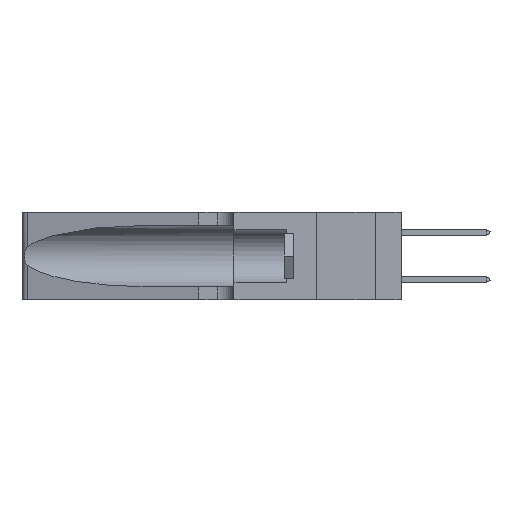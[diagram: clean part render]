
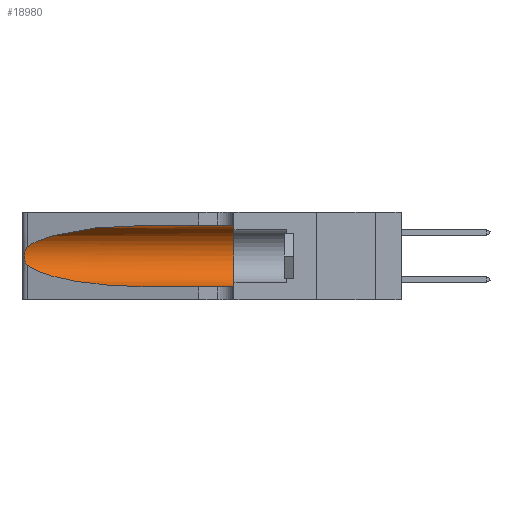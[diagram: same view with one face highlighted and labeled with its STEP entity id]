
A CAD part, left-side view. The second image highlights one B-rep face of the part: STEP entity #18980.
In plain terms, the highlighted cylindrical face has radius 3.308 mm (diameter 6.617 mm), a partial arc.
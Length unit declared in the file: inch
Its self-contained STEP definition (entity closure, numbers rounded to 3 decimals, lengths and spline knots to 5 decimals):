
#847 = CARTESIAN_POINT ( 'NONE',  ( 0.26075, 1.23896, 0.178 ) ) ;
#1594 = B_SPLINE_CURVE_WITH_KNOTS ( 'NONE', 3,
 ( #9400, #29070, #12274, #31901, #15130, #34700, #17978, #847, #20798, #3743, #23626, #6642, #26400, #9530 ),
 .UNSPECIFIED., .F., .F.,
 ( 4, 2, 2, 2, 2, 2, 4 ),
 ( 0., 0.00027, 0.00053, 0.00107, 0.0016, 0.00187, 0.00214 ),
 .UNSPECIFIED. ) ;
#2222 = DIRECTION ( 'NONE',  ( 0., 1., 0. ) ) ;
#2619 = CARTESIAN_POINT ( 'NONE',  ( 0.25487, 1.22718, 0.14631 ) ) ;
#3743 = CARTESIAN_POINT ( 'NONE',  ( 0.25856, 1.23593, 0.16098 ) ) ;
#4929 = LINE ( 'NONE', #19138, #19169 ) ;
#4961 = DIRECTION ( 'NONE',  ( 0., -1., 0. ) ) ;
#5533 =( BOUNDED_CURVE ( )  B_SPLINE_CURVE ( 3, ( #9325, #23425, #15048, #34634 ),
 .UNSPECIFIED., .F., .T. ) 
 B_SPLINE_CURVE_WITH_KNOTS ( ( 4, 4 ),
 ( 3.44316, 4.71239 ),
 .UNSPECIFIED. ) 
 CURVE ( )  GEOMETRIC_REPRESENTATION_ITEM ( )  RATIONAL_B_SPLINE_CURVE ( ( 1., 0.87, 0.87, 1. ) ) 
 REPRESENTATION_ITEM ( '' )  );
#6642 = CARTESIAN_POINT ( 'NONE',  ( 0.25639, 1.23186, 0.15144 ) ) ;
#6939 = CARTESIAN_POINT ( 'NONE',  ( 0.2373, 1.15595, 0.28018 ) ) ;
#7220 = DIRECTION ( 'NONE',  ( 0., -1., 0. ) ) ;
#7723 = AXIS2_PLACEMENT_3D ( 'NONE', #32463, #7220, #26968 ) ;
#7843 = VERTEX_POINT ( 'NONE', #20729 ) ;
#8729 = VERTEX_POINT ( 'NONE', #20618 ) ;
#9325 = CARTESIAN_POINT ( 'NONE',  ( 0.25487, 1.22718, 0.14631 ) ) ;
#9400 = CARTESIAN_POINT ( 'NONE',  ( 0.25487, 1.22718, 0.22369 ) ) ;
#9530 = CARTESIAN_POINT ( 'NONE',  ( 0.25487, 1.22718, 0.14631 ) ) ;
#9717 = CARTESIAN_POINT ( 'NONE',  ( 0.1305, 0.72297, 0.31525 ) ) ;
#12274 = CARTESIAN_POINT ( 'NONE',  ( 0.25639, 1.23184, 0.21858 ) ) ;
#15048 = CARTESIAN_POINT ( 'NONE',  ( 0.18966, 0.96281, 0.05475 ) ) ;
#15130 = CARTESIAN_POINT ( 'NONE',  ( 0.25854, 1.2359, 0.20912 ) ) ;
#16181 = DIRECTION ( 'NONE',  ( 0., -1., 0. ) ) ;
#17978 = CARTESIAN_POINT ( 'NONE',  ( 0.26075, 1.23896, 0.19203 ) ) ;
#18260 = CARTESIAN_POINT ( 'NONE',  ( 0.18966, 0.96281, 0.31525 ) ) ;
#18316 = VERTEX_POINT ( 'NONE', #29688 ) ;
#18980 = ADVANCED_FACE ( 'NONE', ( #30501 ), #22222, .F. ) ;
#19138 = CARTESIAN_POINT ( 'NONE',  ( 0.1305, 1.61858, 0.31525 ) ) ;
#19169 = VECTOR ( 'NONE', #4961, 39.37008 ) ;
#19300 = CARTESIAN_POINT ( 'NONE',  ( 0.1305, 0.35, 0.185 ) ) ;
#20207 = EDGE_CURVE ( 'NONE', #8729, #27805, #1594, .T. ) ;
#20618 = CARTESIAN_POINT ( 'NONE',  ( 0.25487, 1.22718, 0.22369 ) ) ;
#20729 = CARTESIAN_POINT ( 'NONE',  ( 0.1305, 0.72297, 0.05475 ) ) ;
#20798 = CARTESIAN_POINT ( 'NONE',  ( 0.26017, 1.23833, 0.17102 ) ) ;
#20882 = ORIENTED_EDGE ( 'NONE', *, *, #26905, .T. ) ;
#21963 = ORIENTED_EDGE ( 'NONE', *, *, #30637, .T. ) ;
#21986 = ORIENTED_EDGE ( 'NONE', *, *, #20207, .T. ) ;
#22128 = DIRECTION ( 'NONE',  ( 0., 0., 1. ) ) ;
#22222 = CYLINDRICAL_SURFACE ( 'NONE', #7723, 0.13025 ) ;
#23425 = CARTESIAN_POINT ( 'NONE',  ( 0.2373, 1.15595, 0.08982 ) ) ;
#23626 = CARTESIAN_POINT ( 'NONE',  ( 0.25789, 1.23486, 0.15765 ) ) ;
#24091 = VERTEX_POINT ( 'NONE', #27005 ) ;
#24323 = ORIENTED_EDGE ( 'NONE', *, *, #26958, .F. ) ;
#25141 = EDGE_CURVE ( 'NONE', #27805, #7843, #5533, .T. ) ;
#26400 = CARTESIAN_POINT ( 'NONE',  ( 0.25555, 1.22993, 0.14849 ) ) ;
#26703 = CARTESIAN_POINT ( 'NONE',  ( 0.25487, 1.22718, 0.22369 ) ) ;
#26905 = EDGE_CURVE ( 'NONE', #7843, #24091, #28328, .T. ) ;
#26958 = EDGE_CURVE ( 'NONE', #18316, #31938, #4929, .T. ) ;
#26968 = DIRECTION ( 'NONE',  ( 0., 0., -1. ) ) ;
#27005 = CARTESIAN_POINT ( 'NONE',  ( 0.1305, 0.35, 0.05475 ) ) ;
#27805 = VERTEX_POINT ( 'NONE', #2619 ) ;
#27815 = EDGE_LOOP ( 'NONE', ( #21963, #21986, #35365, #20882, #35640, #24323 ) ) ;
#28328 = LINE ( 'NONE', #35726, #31844 ) ;
#29043 =( BOUNDED_CURVE ( )  B_SPLINE_CURVE ( 3, ( #9717, #18260, #6939, #26703 ),
 .UNSPECIFIED., .F., .T. ) 
 B_SPLINE_CURVE_WITH_KNOTS ( ( 4, 4 ),
 ( 1.5708, 2.84003 ),
 .UNSPECIFIED. ) 
 CURVE ( )  GEOMETRIC_REPRESENTATION_ITEM ( )  RATIONAL_B_SPLINE_CURVE ( ( 1., 0.87, 0.87, 1. ) ) 
 REPRESENTATION_ITEM ( '' )  );
#29070 = CARTESIAN_POINT ( 'NONE',  ( 0.25555, 1.22994, 0.2215 ) ) ;
#29688 = CARTESIAN_POINT ( 'NONE',  ( 0.1305, 0.72297, 0.31525 ) ) ;
#30501 = FACE_OUTER_BOUND ( 'NONE', #27815, .T. ) ;
#30637 = EDGE_CURVE ( 'NONE', #18316, #8729, #29043, .T. ) ;
#31844 = VECTOR ( 'NONE', #16181, 39.37008 ) ;
#31901 = CARTESIAN_POINT ( 'NONE',  ( 0.25787, 1.23484, 0.2124 ) ) ;
#31938 = VERTEX_POINT ( 'NONE', #32604 ) ;
#32463 = CARTESIAN_POINT ( 'NONE',  ( 0.1305, 1.61858, 0.185 ) ) ;
#32604 = CARTESIAN_POINT ( 'NONE',  ( 0.1305, 0.35, 0.31525 ) ) ;
#32994 = EDGE_CURVE ( 'NONE', #31938, #24091, #36568, .T. ) ;
#33426 = AXIS2_PLACEMENT_3D ( 'NONE', #19300, #2222, #22128 ) ;
#34634 = CARTESIAN_POINT ( 'NONE',  ( 0.1305, 0.72297, 0.05475 ) ) ;
#34700 = CARTESIAN_POINT ( 'NONE',  ( 0.26018, 1.23835, 0.19895 ) ) ;
#35365 = ORIENTED_EDGE ( 'NONE', *, *, #25141, .T. ) ;
#35640 = ORIENTED_EDGE ( 'NONE', *, *, #32994, .F. ) ;
#35726 = CARTESIAN_POINT ( 'NONE',  ( 0.1305, 1.61858, 0.05475 ) ) ;
#36568 = CIRCLE ( 'NONE', #33426, 0.13025 ) ;
